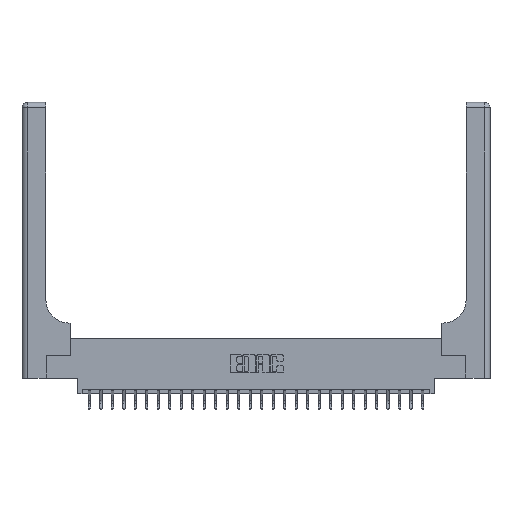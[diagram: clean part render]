
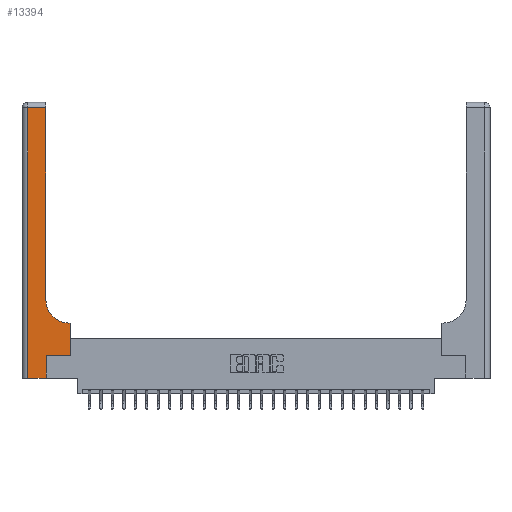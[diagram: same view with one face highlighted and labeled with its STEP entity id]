
A CAD part, top view. The second image highlights one B-rep face of the part: STEP entity #13394.
In plain terms, the highlighted planar face has unit normal (0, 0, 1).
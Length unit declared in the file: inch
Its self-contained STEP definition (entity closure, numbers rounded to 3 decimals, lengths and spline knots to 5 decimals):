
#894 = CARTESIAN_POINT ( 'NONE',  ( 0., 3., 0.37 ) ) ;
#958 = VECTOR ( 'NONE', #3568, 39.37008 ) ;
#1100 = CARTESIAN_POINT ( 'NONE',  ( 0.528, 0.6, 0.37 ) ) ;
#1386 = DIRECTION ( 'NONE',  ( 1., 0., 0. ) ) ;
#1429 = ORIENTED_EDGE ( 'NONE', *, *, #19641, .T. ) ;
#2031 = EDGE_CURVE ( 'NONE', #3830, #19963, #16529, .T. ) ;
#2318 = LINE ( 'NONE', #24364, #18934 ) ;
#2417 = VERTEX_POINT ( 'NONE', #22513 ) ;
#2595 = CARTESIAN_POINT ( 'NONE',  ( 0.528, 0.25, 0.37 ) ) ;
#2827 = VECTOR ( 'NONE', #15092, 39.37008 ) ;
#2871 = DIRECTION ( 'NONE',  ( 0., 1., 0. ) ) ;
#3176 = CARTESIAN_POINT ( 'NONE',  ( 0.06, 3., 0.37 ) ) ;
#3393 = VERTEX_POINT ( 'NONE', #26136 ) ;
#3568 = DIRECTION ( 'NONE',  ( -1., 0., 0. ) ) ;
#3830 = VERTEX_POINT ( 'NONE', #8638 ) ;
#4003 = ORIENTED_EDGE ( 'NONE', *, *, #2031, .T. ) ;
#4077 = CARTESIAN_POINT ( 'NONE',  ( 0.265, 0., 0.37 ) ) ;
#4936 = CIRCLE ( 'NONE', #10865, 0.25 ) ;
#5419 = EDGE_CURVE ( 'NONE', #2417, #20205, #2318, .T. ) ;
#6143 = VECTOR ( 'NONE', #19815, 39.37008 ) ;
#6323 = DIRECTION ( 'NONE',  ( 0., 1., 0. ) ) ;
#6617 = CARTESIAN_POINT ( 'NONE',  ( 0., 2.94, 0.37 ) ) ;
#6631 = ORIENTED_EDGE ( 'NONE', *, *, #10761, .T. ) ;
#7146 = FACE_OUTER_BOUND ( 'NONE', #25310, .T. ) ;
#8582 = ORIENTED_EDGE ( 'NONE', *, *, #5419, .T. ) ;
#8638 = CARTESIAN_POINT ( 'NONE',  ( 0.26, 2.94, 0.37 ) ) ;
#10761 = EDGE_CURVE ( 'NONE', #15206, #2417, #11863, .T. ) ;
#10865 = AXIS2_PLACEMENT_3D ( 'NONE', #26137, #13874, #1386 ) ;
#11355 = VERTEX_POINT ( 'NONE', #17326 ) ;
#11372 = DIRECTION ( 'NONE',  ( 0., 0., -1. ) ) ;
#11863 = LINE ( 'NONE', #15359, #17376 ) ;
#12158 = VECTOR ( 'NONE', #6323, 39.37008 ) ;
#13394 = ADVANCED_FACE ( 'NONE', ( #7146 ), #21660, .F. ) ;
#13874 = DIRECTION ( 'NONE',  ( 0., 0., -1. ) ) ;
#13964 = CARTESIAN_POINT ( 'NONE',  ( 0.26, 0.6, 0.37 ) ) ;
#14146 = DIRECTION ( 'NONE',  ( 1., 0., 0. ) ) ;
#14616 = CARTESIAN_POINT ( 'NONE',  ( 0.26, 3., 0.37 ) ) ;
#14650 = DIRECTION ( 'NONE',  ( 1., 0., 0. ) ) ;
#14739 = VERTEX_POINT ( 'NONE', #1100 ) ;
#15092 = DIRECTION ( 'NONE',  ( 0., 1., 0. ) ) ;
#15206 = VERTEX_POINT ( 'NONE', #4077 ) ;
#15359 = CARTESIAN_POINT ( 'NONE',  ( 0.265, 0., 0.37 ) ) ;
#15615 = AXIS2_PLACEMENT_3D ( 'NONE', #894, #11372, #25742 ) ;
#16099 = LINE ( 'NONE', #16660, #20920 ) ;
#16529 = LINE ( 'NONE', #6617, #26095 ) ;
#16660 = CARTESIAN_POINT ( 'NONE',  ( 0., 0., 0.37 ) ) ;
#16983 = DIRECTION ( 'NONE',  ( -1., 0., 0. ) ) ;
#17012 = LINE ( 'NONE', #14616, #12158 ) ;
#17043 = ORIENTED_EDGE ( 'NONE', *, *, #17895, .T. ) ;
#17326 = CARTESIAN_POINT ( 'NONE',  ( 0.26, 0.85, 0.37 ) ) ;
#17376 = VECTOR ( 'NONE', #2871, 39.37008 ) ;
#17895 = EDGE_CURVE ( 'NONE', #25774, #15206, #16099, .T. ) ;
#18012 = CARTESIAN_POINT ( 'NONE',  ( 0.528, 0.25, 0.37 ) ) ;
#18934 = VECTOR ( 'NONE', #14146, 39.37008 ) ;
#19282 = EDGE_CURVE ( 'NONE', #11355, #3830, #17012, .T. ) ;
#19641 = EDGE_CURVE ( 'NONE', #3393, #11355, #4936, .T. ) ;
#19815 = DIRECTION ( 'NONE',  ( 0., -1., 0. ) ) ;
#19963 = VERTEX_POINT ( 'NONE', #23540 ) ;
#20205 = VERTEX_POINT ( 'NONE', #18012 ) ;
#20269 = ORIENTED_EDGE ( 'NONE', *, *, #24732, .T. ) ;
#20676 = EDGE_CURVE ( 'NONE', #14739, #3393, #22367, .T. ) ;
#20905 = ORIENTED_EDGE ( 'NONE', *, *, #20676, .T. ) ;
#20920 = VECTOR ( 'NONE', #14650, 39.37008 ) ;
#21153 = ORIENTED_EDGE ( 'NONE', *, *, #19282, .T. ) ;
#21660 = PLANE ( 'NONE',  #15615 ) ;
#22367 = LINE ( 'NONE', #13964, #958 ) ;
#22513 = CARTESIAN_POINT ( 'NONE',  ( 0.265, 0.25, 0.37 ) ) ;
#23275 = LINE ( 'NONE', #3176, #6143 ) ;
#23540 = CARTESIAN_POINT ( 'NONE',  ( 0.06, 2.94, 0.37 ) ) ;
#24236 = EDGE_CURVE ( 'NONE', #19963, #25774, #23275, .T. ) ;
#24364 = CARTESIAN_POINT ( 'NONE',  ( 0.265, 0.25, 0.37 ) ) ;
#24732 = EDGE_CURVE ( 'NONE', #20205, #14739, #24833, .T. ) ;
#24833 = LINE ( 'NONE', #2595, #2827 ) ;
#25310 = EDGE_LOOP ( 'NONE', ( #21153, #4003, #26623, #17043, #6631, #8582, #20269, #20905, #1429 ) ) ;
#25742 = DIRECTION ( 'NONE',  ( -1., 0., 0. ) ) ;
#25774 = VERTEX_POINT ( 'NONE', #26576 ) ;
#26095 = VECTOR ( 'NONE', #16983, 39.37008 ) ;
#26136 = CARTESIAN_POINT ( 'NONE',  ( 0.51, 0.6, 0.37 ) ) ;
#26137 = CARTESIAN_POINT ( 'NONE',  ( 0.51, 0.85, 0.37 ) ) ;
#26576 = CARTESIAN_POINT ( 'NONE',  ( 0.06, 0., 0.37 ) ) ;
#26623 = ORIENTED_EDGE ( 'NONE', *, *, #24236, .T. ) ;
